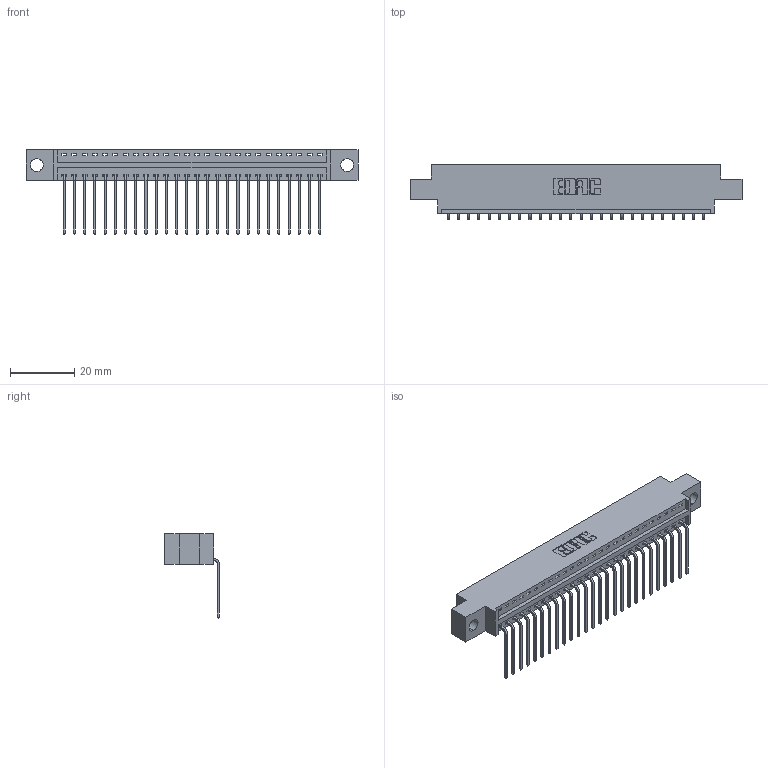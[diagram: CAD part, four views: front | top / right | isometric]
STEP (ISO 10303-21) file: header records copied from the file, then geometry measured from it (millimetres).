
FILE_DESCRIPTION (( 'STEP AP203' ), '1' );
FILE_NAME ('346-026-559-604.STEP', '2022-05-06T03:40:18', ( '' ), ( '' ), 'SwSTEP 2.0', 'SolidWorks 2020', '' );
FILE_SCHEMA (( 'CONFIG_CONTROL_DESIGN' ));
Length unit declared in the file: inch
Products named in the file (3): 346 Part_0.170 Offset - 0.156 Dia-TH; 345-292-001_558 559 Tail - 1; 346-026-559-604
Assembly tree (27 placements, depth 2):
  346-026-559-604
    346 Part_0.170 Offset - 0.156 Dia-TH
    345-292-001_558 559 Tail - 1  x26
Bounding box: 103.12 x 17.08 x 26.16 mm (x, y, z)
Volume: 9587.1 mm3; surface area: 12324.3 mm2
Topology: 27 solids, 27 shells, 1700 faces, 5109 edges, 3370 vertices
Faces by surface type: plane 1186, cylinder 514
Entity records: 18925 total; most frequent: CARTESIAN_POINT 3260, ORIENTED_EDGE 3218, DIRECTION 2893, EDGE_CURVE 1609, LINE 1373, VECTOR 1373, VERTEX_POINT 1070, AXIS2_PLACEMENT_3D 760
